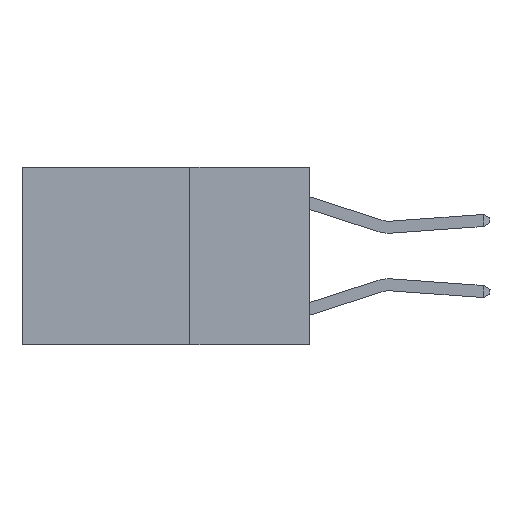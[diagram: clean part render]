
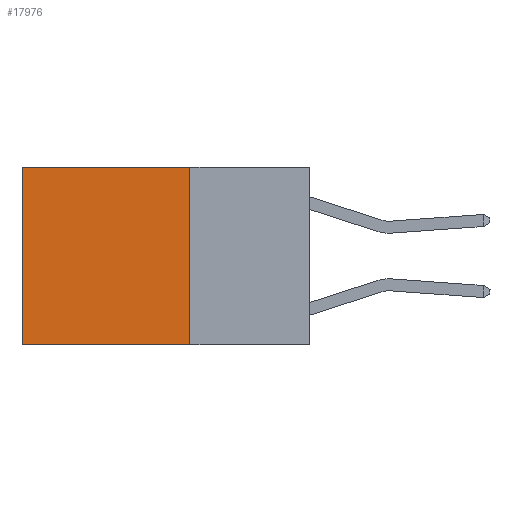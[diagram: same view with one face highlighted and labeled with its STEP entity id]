
A CAD part, left-side view. The second image highlights one B-rep face of the part: STEP entity #17976.
In plain terms, the highlighted planar face has unit normal (-1, 0, 0).
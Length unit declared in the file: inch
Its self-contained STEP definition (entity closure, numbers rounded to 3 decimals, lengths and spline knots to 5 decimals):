
#472 = EDGE_CURVE ( 'NONE', #12293, #13916, #29797, .T. ) ;
#996 = VECTOR ( 'NONE', #32697, 39.37008 ) ;
#2481 = CARTESIAN_POINT ( 'NONE',  ( 0.2625, 0.25, 0. ) ) ;
#3613 = VECTOR ( 'NONE', #20409, 39.37008 ) ;
#3646 = EDGE_LOOP ( 'NONE', ( #14554, #12070, #27040, #19128 ) ) ;
#3872 = DIRECTION ( 'NONE',  ( 0., 0., -1. ) ) ;
#8413 = CARTESIAN_POINT ( 'NONE',  ( 0.2625, 0.25, 0. ) ) ;
#8916 = CARTESIAN_POINT ( 'NONE',  ( 0.2625, 0.25, 0. ) ) ;
#9997 = VERTEX_POINT ( 'NONE', #19701 ) ;
#10316 = FACE_OUTER_BOUND ( 'NONE', #3646, .T. ) ;
#11676 = EDGE_CURVE ( 'NONE', #11762, #9997, #11721, .T. ) ;
#11721 = LINE ( 'NONE', #28940, #24432 ) ;
#11762 = VERTEX_POINT ( 'NONE', #24146 ) ;
#12070 = ORIENTED_EDGE ( 'NONE', *, *, #24320, .F. ) ;
#12293 = VERTEX_POINT ( 'NONE', #8413 ) ;
#13916 = VERTEX_POINT ( 'NONE', #17373 ) ;
#14037 = PLANE ( 'NONE',  #30194 ) ;
#14509 = LINE ( 'NONE', #26680, #20519 ) ;
#14554 = ORIENTED_EDGE ( 'NONE', *, *, #11676, .T. ) ;
#17373 = CARTESIAN_POINT ( 'NONE',  ( 0.2625, 0.25, -0.37 ) ) ;
#17976 = ADVANCED_FACE ( 'NONE', ( #10316 ), #14037, .F. ) ;
#19128 = ORIENTED_EDGE ( 'NONE', *, *, #22629, .T. ) ;
#19187 = DIRECTION ( 'NONE',  ( 1., 0., 0. ) ) ;
#19701 = CARTESIAN_POINT ( 'NONE',  ( 0.2625, 0.6, -0.37 ) ) ;
#20409 = DIRECTION ( 'NONE',  ( 0., 0., -1. ) ) ;
#20519 = VECTOR ( 'NONE', #31675, 39.37008 ) ;
#20645 = LINE ( 'NONE', #25211, #996 ) ;
#22629 = EDGE_CURVE ( 'NONE', #12293, #11762, #20645, .T. ) ;
#24146 = CARTESIAN_POINT ( 'NONE',  ( 0.2625, 0.6, 0. ) ) ;
#24320 = EDGE_CURVE ( 'NONE', #13916, #9997, #14509, .T. ) ;
#24432 = VECTOR ( 'NONE', #26439, 39.37008 ) ;
#25211 = CARTESIAN_POINT ( 'NONE',  ( 0.2625, 0.25, 0. ) ) ;
#26439 = DIRECTION ( 'NONE',  ( 0., 0., -1. ) ) ;
#26680 = CARTESIAN_POINT ( 'NONE',  ( 0.2625, 0.25, -0.37 ) ) ;
#27040 = ORIENTED_EDGE ( 'NONE', *, *, #472, .F. ) ;
#28940 = CARTESIAN_POINT ( 'NONE',  ( 0.2625, 0.6, 0. ) ) ;
#29797 = LINE ( 'NONE', #2481, #3613 ) ;
#30194 = AXIS2_PLACEMENT_3D ( 'NONE', #8916, #19187, #3872 ) ;
#31675 = DIRECTION ( 'NONE',  ( 0., 1., 0. ) ) ;
#32697 = DIRECTION ( 'NONE',  ( 0., 1., 0. ) ) ;
